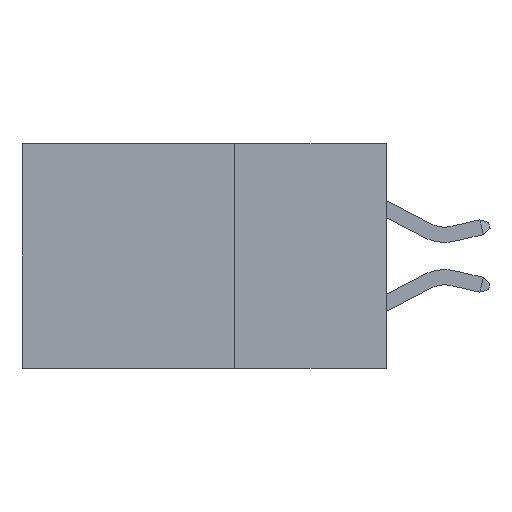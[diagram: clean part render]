
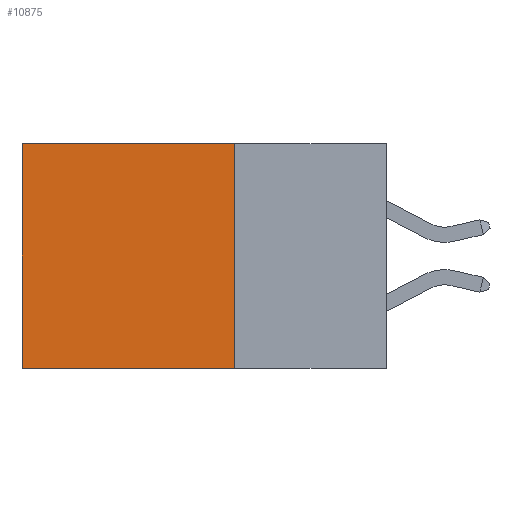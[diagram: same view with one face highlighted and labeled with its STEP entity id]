
A CAD part, left-side view. The second image highlights one B-rep face of the part: STEP entity #10875.
In plain terms, the highlighted planar face has unit normal (-1, 0, 0).
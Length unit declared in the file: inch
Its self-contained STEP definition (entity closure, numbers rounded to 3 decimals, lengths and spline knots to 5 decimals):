
#1532 = CARTESIAN_POINT ( 'NONE',  ( 0.298, 0.25, 0. ) ) ;
#1827 = VERTEX_POINT ( 'NONE', #10873 ) ;
#1888 = EDGE_LOOP ( 'NONE', ( #9054, #3552, #5776, #10092 ) ) ;
#2569 = DIRECTION ( 'NONE',  ( 0., 1., 0. ) ) ;
#2912 = LINE ( 'NONE', #1532, #5352 ) ;
#3318 = CARTESIAN_POINT ( 'NONE',  ( 0.298, 0.25, -0.37 ) ) ;
#3421 = VERTEX_POINT ( 'NONE', #3318 ) ;
#3552 = ORIENTED_EDGE ( 'NONE', *, *, #8422, .F. ) ;
#4860 = CARTESIAN_POINT ( 'NONE',  ( 0.298, 0.25, 0. ) ) ;
#5352 = VECTOR ( 'NONE', #2569, 39.37008 ) ;
#5675 = VECTOR ( 'NONE', #8784, 39.37008 ) ;
#5752 = CARTESIAN_POINT ( 'NONE',  ( 0.298, 0.25, 0. ) ) ;
#5776 = ORIENTED_EDGE ( 'NONE', *, *, #11489, .F. ) ;
#5823 = VECTOR ( 'NONE', #6628, 39.37008 ) ;
#5869 = DIRECTION ( 'NONE',  ( 0., 0., -1. ) ) ;
#6146 = FACE_OUTER_BOUND ( 'NONE', #1888, .T. ) ;
#6212 = LINE ( 'NONE', #6834, #10606 ) ;
#6628 = DIRECTION ( 'NONE',  ( 0., 0., -1. ) ) ;
#6782 = CARTESIAN_POINT ( 'NONE',  ( 0.298, 0.6, -0.37 ) ) ;
#6834 = CARTESIAN_POINT ( 'NONE',  ( 0.298, 0.25, -0.37 ) ) ;
#7796 = DIRECTION ( 'NONE',  ( 0., 1., 0. ) ) ;
#8229 = LINE ( 'NONE', #9708, #5675 ) ;
#8327 = VERTEX_POINT ( 'NONE', #5752 ) ;
#8386 = LINE ( 'NONE', #8511, #5823 ) ;
#8422 = EDGE_CURVE ( 'NONE', #3421, #9002, #6212, .T. ) ;
#8511 = CARTESIAN_POINT ( 'NONE',  ( 0.298, 0.6, 0. ) ) ;
#8784 = DIRECTION ( 'NONE',  ( 0., 0., -1. ) ) ;
#9002 = VERTEX_POINT ( 'NONE', #6782 ) ;
#9054 = ORIENTED_EDGE ( 'NONE', *, *, #11275, .T. ) ;
#9708 = CARTESIAN_POINT ( 'NONE',  ( 0.298, 0.25, 0. ) ) ;
#10092 = ORIENTED_EDGE ( 'NONE', *, *, #11917, .T. ) ;
#10554 = PLANE ( 'NONE',  #11034 ) ;
#10606 = VECTOR ( 'NONE', #7796, 39.37008 ) ;
#10873 = CARTESIAN_POINT ( 'NONE',  ( 0.298, 0.6, 0. ) ) ;
#10875 = ADVANCED_FACE ( 'NONE', ( #6146 ), #10554, .F. ) ;
#11034 = AXIS2_PLACEMENT_3D ( 'NONE', #4860, #11484, #5869 ) ;
#11275 = EDGE_CURVE ( 'NONE', #1827, #9002, #8386, .T. ) ;
#11484 = DIRECTION ( 'NONE',  ( 1., 0., 0. ) ) ;
#11489 = EDGE_CURVE ( 'NONE', #8327, #3421, #8229, .T. ) ;
#11917 = EDGE_CURVE ( 'NONE', #8327, #1827, #2912, .T. ) ;
